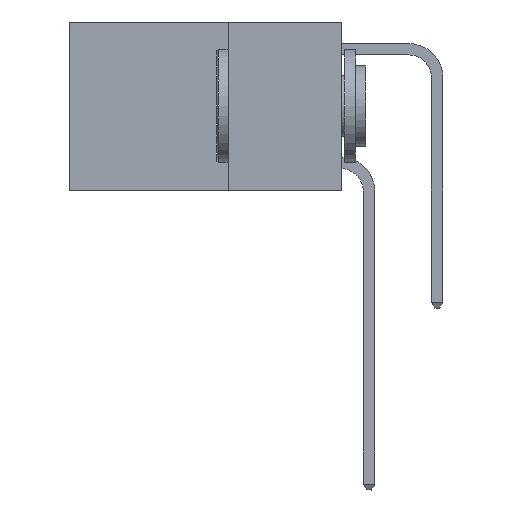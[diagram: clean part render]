
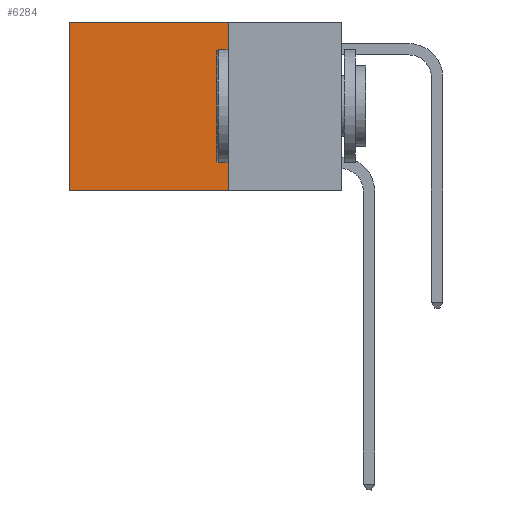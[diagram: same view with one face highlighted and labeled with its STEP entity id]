
A CAD part, left-side view. The second image highlights one B-rep face of the part: STEP entity #6284.
In plain terms, the highlighted planar face has unit normal (-1, 0, 0).
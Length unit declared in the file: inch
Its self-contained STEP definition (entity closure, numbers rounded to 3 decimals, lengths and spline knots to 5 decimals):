
#1805 = DIRECTION ( 'NONE',  ( 0., 0., -1. ) ) ;
#1877 = CARTESIAN_POINT ( 'NONE',  ( 0.2625, 0.25, 0. ) ) ;
#3336 = ORIENTED_EDGE ( 'NONE', *, *, #7246, .F. ) ;
#3485 = VECTOR ( 'NONE', #9576, 39.37008 ) ;
#5585 = VECTOR ( 'NONE', #21067, 39.37008 ) ;
#6284 = ADVANCED_FACE ( 'NONE', ( #22905 ), #11822, .F. ) ;
#6944 = LINE ( 'NONE', #11697, #5585 ) ;
#7246 = EDGE_CURVE ( 'NONE', #18845, #12200, #22829, .T. ) ;
#7727 = VECTOR ( 'NONE', #1805, 39.37008 ) ;
#7745 = CARTESIAN_POINT ( 'NONE',  ( 0.2625, 0.25, -0.37 ) ) ;
#9576 = DIRECTION ( 'NONE',  ( 0., 1., 0. ) ) ;
#10535 = CARTESIAN_POINT ( 'NONE',  ( 0.2625, 0.25, 0. ) ) ;
#10547 = VERTEX_POINT ( 'NONE', #24690 ) ;
#11487 = ORIENTED_EDGE ( 'NONE', *, *, #21465, .T. ) ;
#11697 = CARTESIAN_POINT ( 'NONE',  ( 0.2625, 0.6, 0. ) ) ;
#11822 = PLANE ( 'NONE',  #12566 ) ;
#12200 = VERTEX_POINT ( 'NONE', #7745 ) ;
#12241 = CARTESIAN_POINT ( 'NONE',  ( 0.2625, 0.25, 0. ) ) ;
#12566 = AXIS2_PLACEMENT_3D ( 'NONE', #1877, #27951, #20750 ) ;
#14876 = CARTESIAN_POINT ( 'NONE',  ( 0.2625, 0.6, 0. ) ) ;
#16252 = DIRECTION ( 'NONE',  ( 0., 1., 0. ) ) ;
#16701 = LINE ( 'NONE', #12241, #26534 ) ;
#17496 = ORIENTED_EDGE ( 'NONE', *, *, #22452, .F. ) ;
#17845 = ORIENTED_EDGE ( 'NONE', *, *, #24482, .T. ) ;
#18845 = VERTEX_POINT ( 'NONE', #10535 ) ;
#20750 = DIRECTION ( 'NONE',  ( 0., 0., -1. ) ) ;
#21067 = DIRECTION ( 'NONE',  ( 0., 0., -1. ) ) ;
#21465 = EDGE_CURVE ( 'NONE', #25968, #10547, #6944, .T. ) ;
#21725 = CARTESIAN_POINT ( 'NONE',  ( 0.2625, 0.25, -0.37 ) ) ;
#22452 = EDGE_CURVE ( 'NONE', #12200, #10547, #28321, .T. ) ;
#22829 = LINE ( 'NONE', #23273, #7727 ) ;
#22905 = FACE_OUTER_BOUND ( 'NONE', #23069, .T. ) ;
#23069 = EDGE_LOOP ( 'NONE', ( #11487, #17496, #3336, #17845 ) ) ;
#23273 = CARTESIAN_POINT ( 'NONE',  ( 0.2625, 0.25, 0. ) ) ;
#24482 = EDGE_CURVE ( 'NONE', #18845, #25968, #16701, .T. ) ;
#24690 = CARTESIAN_POINT ( 'NONE',  ( 0.2625, 0.6, -0.37 ) ) ;
#25968 = VERTEX_POINT ( 'NONE', #14876 ) ;
#26534 = VECTOR ( 'NONE', #16252, 39.37008 ) ;
#27951 = DIRECTION ( 'NONE',  ( 1., 0., 0. ) ) ;
#28321 = LINE ( 'NONE', #21725, #3485 ) ;
